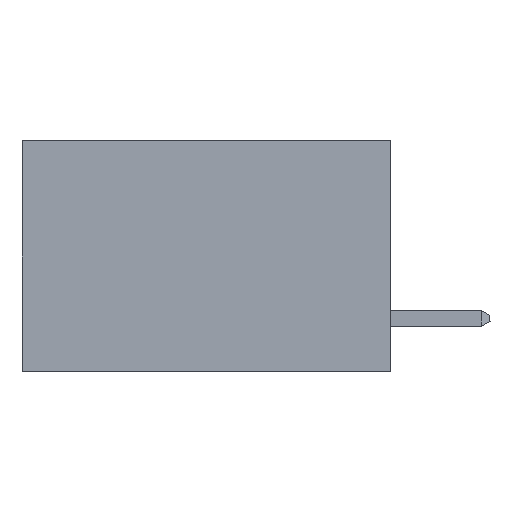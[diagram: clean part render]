
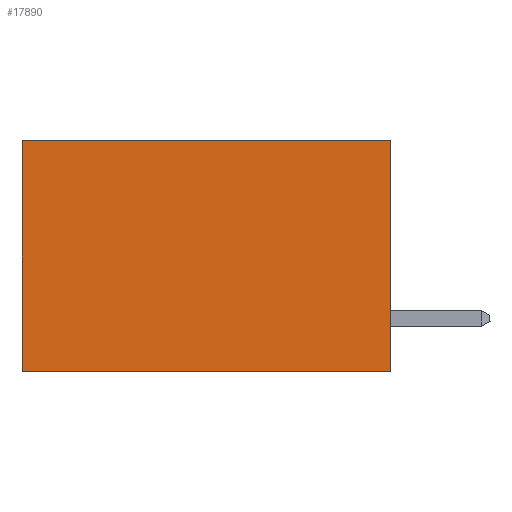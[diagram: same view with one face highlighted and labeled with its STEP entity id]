
A CAD part, left-side view. The second image highlights one B-rep face of the part: STEP entity #17890.
In plain terms, the highlighted planar face has unit normal (-1, 0, 0).
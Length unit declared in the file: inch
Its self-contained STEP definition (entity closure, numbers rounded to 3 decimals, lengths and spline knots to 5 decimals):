
#44 = DIRECTION ( 'NONE',  ( 1., 0., 0. ) ) ;
#195 = EDGE_CURVE ( 'NONE', #20808, #10656, #9000, .T. ) ;
#431 = ORIENTED_EDGE ( 'NONE', *, *, #27611, .T. ) ;
#1222 = CARTESIAN_POINT ( 'NONE',  ( 0.277, 0.59, -0.37 ) ) ;
#2777 = ORIENTED_EDGE ( 'NONE', *, *, #195, .F. ) ;
#2943 = EDGE_LOOP ( 'NONE', ( #431, #2777, #3535, #11698 ) ) ;
#3143 = VECTOR ( 'NONE', #22801, 39.37008 ) ;
#3535 = ORIENTED_EDGE ( 'NONE', *, *, #4942, .F. ) ;
#4581 = CARTESIAN_POINT ( 'NONE',  ( 0.277, 0.59, 0. ) ) ;
#4920 = VECTOR ( 'NONE', #14513, 39.37008 ) ;
#4942 = EDGE_CURVE ( 'NONE', #9513, #20808, #13424, .T. ) ;
#4995 = CARTESIAN_POINT ( 'NONE',  ( 0.277, 0., -0.37 ) ) ;
#6203 = CARTESIAN_POINT ( 'NONE',  ( 0.277, 0., 0. ) ) ;
#6423 = CARTESIAN_POINT ( 'NONE',  ( 0.277, 0.59, -0.37 ) ) ;
#7620 = VECTOR ( 'NONE', #25561, 39.37008 ) ;
#9000 = LINE ( 'NONE', #4995, #3143 ) ;
#9513 = VERTEX_POINT ( 'NONE', #6203 ) ;
#10656 = VERTEX_POINT ( 'NONE', #1222 ) ;
#10687 = EDGE_CURVE ( 'NONE', #9513, #24176, #27990, .T. ) ;
#11617 = FACE_OUTER_BOUND ( 'NONE', #2943, .T. ) ;
#11698 = ORIENTED_EDGE ( 'NONE', *, *, #10687, .T. ) ;
#12300 = CARTESIAN_POINT ( 'NONE',  ( 0.277, 0., 0. ) ) ;
#13232 = CARTESIAN_POINT ( 'NONE',  ( 0.277, 0., -0.37 ) ) ;
#13424 = LINE ( 'NONE', #25830, #7620 ) ;
#14513 = DIRECTION ( 'NONE',  ( 0., 1., 0. ) ) ;
#15474 = DIRECTION ( 'NONE',  ( 0., 0., -1. ) ) ;
#17890 = ADVANCED_FACE ( 'NONE', ( #11617 ), #24010, .F. ) ;
#18069 = VECTOR ( 'NONE', #23819, 39.37008 ) ;
#18727 = LINE ( 'NONE', #6423, #18069 ) ;
#20808 = VERTEX_POINT ( 'NONE', #26976 ) ;
#22476 = AXIS2_PLACEMENT_3D ( 'NONE', #13232, #44, #15474 ) ;
#22801 = DIRECTION ( 'NONE',  ( 0., 1., 0. ) ) ;
#23819 = DIRECTION ( 'NONE',  ( 0., 0., -1. ) ) ;
#24010 = PLANE ( 'NONE',  #22476 ) ;
#24176 = VERTEX_POINT ( 'NONE', #4581 ) ;
#25561 = DIRECTION ( 'NONE',  ( 0., 0., -1. ) ) ;
#25830 = CARTESIAN_POINT ( 'NONE',  ( 0.277, 0., -0.37 ) ) ;
#26976 = CARTESIAN_POINT ( 'NONE',  ( 0.277, 0., -0.37 ) ) ;
#27611 = EDGE_CURVE ( 'NONE', #24176, #10656, #18727, .T. ) ;
#27990 = LINE ( 'NONE', #12300, #4920 ) ;
